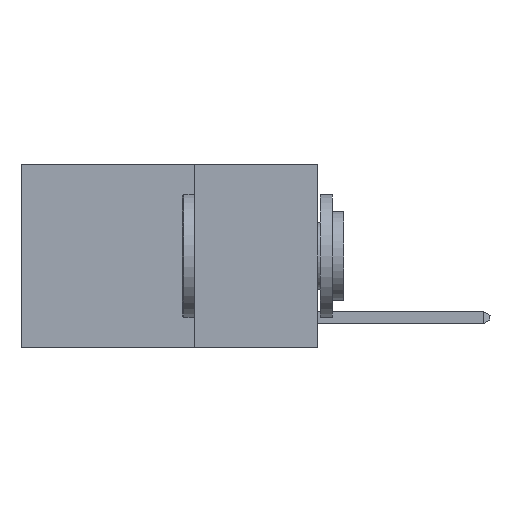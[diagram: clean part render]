
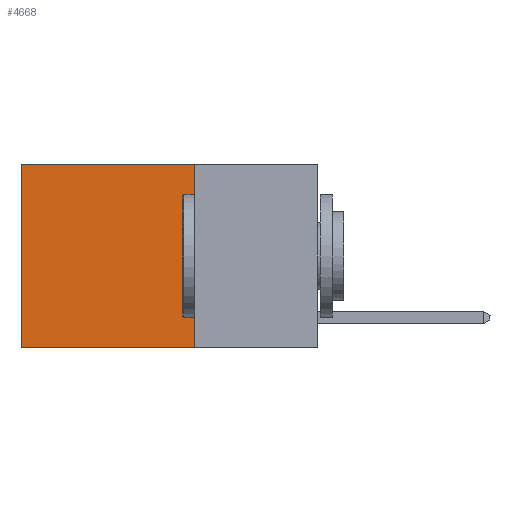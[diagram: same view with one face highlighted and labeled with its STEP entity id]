
A CAD part, left-side view. The second image highlights one B-rep face of the part: STEP entity #4668.
In plain terms, the highlighted planar face has unit normal (-1, 0, 0).
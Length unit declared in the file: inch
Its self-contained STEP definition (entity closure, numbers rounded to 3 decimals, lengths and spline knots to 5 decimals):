
#325 = CARTESIAN_POINT ( 'NONE',  ( 0.2625, 0.25, 0. ) ) ;
#1319 = LINE ( 'NONE', #6514, #14010 ) ;
#2820 = EDGE_CURVE ( 'NONE', #11814, #5469, #9369, .T. ) ;
#2848 = CARTESIAN_POINT ( 'NONE',  ( 0.2625, 0.6, 0. ) ) ;
#3273 = CARTESIAN_POINT ( 'NONE',  ( 0.2625, 0.25, 0. ) ) ;
#3431 = ORIENTED_EDGE ( 'NONE', *, *, #2820, .F. ) ;
#3517 = LINE ( 'NONE', #6225, #11611 ) ;
#3994 = FACE_OUTER_BOUND ( 'NONE', #7759, .T. ) ;
#3998 = PLANE ( 'NONE',  #14193 ) ;
#4283 = CARTESIAN_POINT ( 'NONE',  ( 0.2625, 0.25, -0.37 ) ) ;
#4627 = VERTEX_POINT ( 'NONE', #2848 ) ;
#4668 = ADVANCED_FACE ( 'NONE', ( #3994 ), #3998, .F. ) ;
#4820 = ORIENTED_EDGE ( 'NONE', *, *, #13048, .T. ) ;
#5414 = VECTOR ( 'NONE', #13331, 39.37008 ) ;
#5469 = VERTEX_POINT ( 'NONE', #4283 ) ;
#5861 = EDGE_CURVE ( 'NONE', #5469, #13049, #1319, .T. ) ;
#6222 = DIRECTION ( 'NONE',  ( 0., 1., 0. ) ) ;
#6225 = CARTESIAN_POINT ( 'NONE',  ( 0.2625, 0.6, 0. ) ) ;
#6391 = VECTOR ( 'NONE', #9605, 39.37008 ) ;
#6514 = CARTESIAN_POINT ( 'NONE',  ( 0.2625, 0.25, -0.37 ) ) ;
#7759 = EDGE_LOOP ( 'NONE', ( #14057, #10069, #3431, #4820 ) ) ;
#7876 = CARTESIAN_POINT ( 'NONE',  ( 0.2625, 0.6, -0.37 ) ) ;
#9369 = LINE ( 'NONE', #14051, #6391 ) ;
#9605 = DIRECTION ( 'NONE',  ( 0., 0., -1. ) ) ;
#9704 = DIRECTION ( 'NONE',  ( 0., 0., -1. ) ) ;
#10069 = ORIENTED_EDGE ( 'NONE', *, *, #5861, .F. ) ;
#11489 = EDGE_CURVE ( 'NONE', #4627, #13049, #3517, .T. ) ;
#11611 = VECTOR ( 'NONE', #14157, 39.37008 ) ;
#11814 = VERTEX_POINT ( 'NONE', #325 ) ;
#11889 = DIRECTION ( 'NONE',  ( 1., 0., 0. ) ) ;
#12477 = LINE ( 'NONE', #3273, #5414 ) ;
#13048 = EDGE_CURVE ( 'NONE', #11814, #4627, #12477, .T. ) ;
#13049 = VERTEX_POINT ( 'NONE', #7876 ) ;
#13331 = DIRECTION ( 'NONE',  ( 0., 1., 0. ) ) ;
#14010 = VECTOR ( 'NONE', #6222, 39.37008 ) ;
#14051 = CARTESIAN_POINT ( 'NONE',  ( 0.2625, 0.25, 0. ) ) ;
#14057 = ORIENTED_EDGE ( 'NONE', *, *, #11489, .T. ) ;
#14157 = DIRECTION ( 'NONE',  ( 0., 0., -1. ) ) ;
#14193 = AXIS2_PLACEMENT_3D ( 'NONE', #14196, #11889, #9704 ) ;
#14196 = CARTESIAN_POINT ( 'NONE',  ( 0.2625, 0.25, 0. ) ) ;
